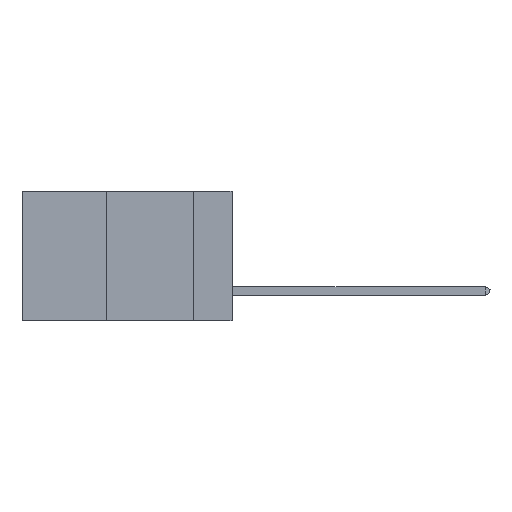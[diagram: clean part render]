
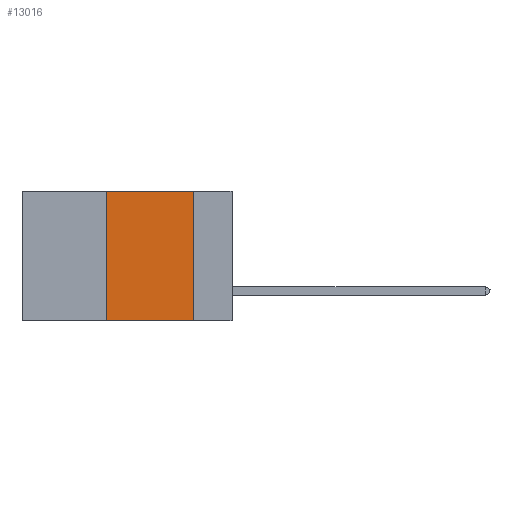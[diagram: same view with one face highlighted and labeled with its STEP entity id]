
A CAD part, left-side view. The second image highlights one B-rep face of the part: STEP entity #13016.
In plain terms, the highlighted planar face has unit normal (-1, 0, 0).
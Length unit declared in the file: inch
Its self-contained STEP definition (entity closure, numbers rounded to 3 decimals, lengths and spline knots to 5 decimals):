
#1524 = CARTESIAN_POINT ( 'NONE',  ( 0., 0.36, -0.37 ) ) ;
#2630 = FACE_OUTER_BOUND ( 'NONE', #20865, .T. ) ;
#6587 = CARTESIAN_POINT ( 'NONE',  ( 0., 0.6, 0. ) ) ;
#7162 = AXIS2_PLACEMENT_3D ( 'NONE', #23760, #26651, #11966 ) ;
#7168 = LINE ( 'NONE', #26682, #24209 ) ;
#7436 = ORIENTED_EDGE ( 'NONE', *, *, #12015, .F. ) ;
#7640 = VECTOR ( 'NONE', #14468, 39.37008 ) ;
#8474 = CARTESIAN_POINT ( 'NONE',  ( 0., 0.11, 0. ) ) ;
#10851 = ORIENTED_EDGE ( 'NONE', *, *, #21505, .T. ) ;
#10994 = ORIENTED_EDGE ( 'NONE', *, *, #36977, .F. ) ;
#11966 = DIRECTION ( 'NONE',  ( 0., 0., -1. ) ) ;
#12015 = EDGE_CURVE ( 'NONE', #23773, #32551, #7168, .T. ) ;
#12537 = LINE ( 'NONE', #8474, #7640 ) ;
#12650 = VERTEX_POINT ( 'NONE', #36090 ) ;
#13016 = ADVANCED_FACE ( 'NONE', ( #2630 ), #20606, .F. ) ;
#14468 = DIRECTION ( 'NONE',  ( 0., 0., -1. ) ) ;
#19132 = VERTEX_POINT ( 'NONE', #23848 ) ;
#19428 = LINE ( 'NONE', #34645, #26179 ) ;
#20606 = PLANE ( 'NONE',  #7162 ) ;
#20865 = EDGE_LOOP ( 'NONE', ( #10994, #24149, #7436, #10851 ) ) ;
#21004 = VECTOR ( 'NONE', #23319, 39.37008 ) ;
#21505 = EDGE_CURVE ( 'NONE', #23773, #12650, #19428, .T. ) ;
#23319 = DIRECTION ( 'NONE',  ( 0., -1., 0. ) ) ;
#23741 = CARTESIAN_POINT ( 'NONE',  ( 0., 0.36, 0. ) ) ;
#23760 = CARTESIAN_POINT ( 'NONE',  ( 0., 0.6, 0. ) ) ;
#23773 = VERTEX_POINT ( 'NONE', #1524 ) ;
#23848 = CARTESIAN_POINT ( 'NONE',  ( 0., 0.11, 0. ) ) ;
#24149 = ORIENTED_EDGE ( 'NONE', *, *, #28360, .F. ) ;
#24209 = VECTOR ( 'NONE', #29689, 39.37008 ) ;
#24233 = DIRECTION ( 'NONE',  ( 0., -1., 0. ) ) ;
#26179 = VECTOR ( 'NONE', #24233, 39.37008 ) ;
#26651 = DIRECTION ( 'NONE',  ( 1., 0., 0. ) ) ;
#26682 = CARTESIAN_POINT ( 'NONE',  ( 0., 0.36, 0. ) ) ;
#28360 = EDGE_CURVE ( 'NONE', #32551, #19132, #30024, .T. ) ;
#29689 = DIRECTION ( 'NONE',  ( 0., 0., 1. ) ) ;
#30024 = LINE ( 'NONE', #6587, #21004 ) ;
#32551 = VERTEX_POINT ( 'NONE', #23741 ) ;
#34645 = CARTESIAN_POINT ( 'NONE',  ( 0., 0.6, -0.37 ) ) ;
#36090 = CARTESIAN_POINT ( 'NONE',  ( 0., 0.11, -0.37 ) ) ;
#36977 = EDGE_CURVE ( 'NONE', #19132, #12650, #12537, .T. ) ;
